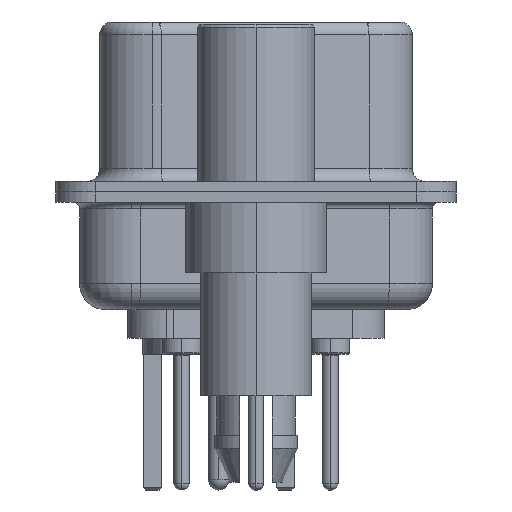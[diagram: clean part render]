
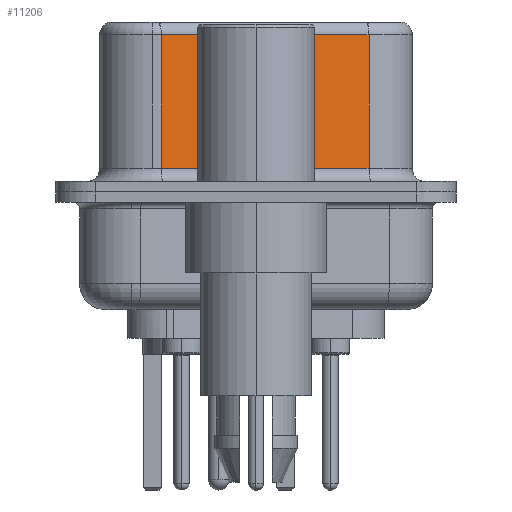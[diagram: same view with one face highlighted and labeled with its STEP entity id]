
A CAD part, left-side view. The second image highlights one B-rep face of the part: STEP entity #11206.
In plain terms, the highlighted planar face has unit normal (-0.985, -0.174, 0).
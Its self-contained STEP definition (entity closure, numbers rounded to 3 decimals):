
#1480 = ORIENTED_EDGE ( 'NONE', *, *, #23325, .T. ) ;
#1945 = VERTEX_POINT ( 'NONE', #15539 ) ;
#2792 = DIRECTION ( 'NONE',  ( 0.174, -0.985, 0. ) ) ;
#2866 = ORIENTED_EDGE ( 'NONE', *, *, #33034, .F. ) ;
#4109 = VERTEX_POINT ( 'NONE', #19650 ) ;
#4393 = CARTESIAN_POINT ( 'NONE',  ( 5.132, -4.322, 6.02 ) ) ;
#5450 = FACE_OUTER_BOUND ( 'NONE', #17898, .T. ) ;
#7857 = LINE ( 'NONE', #10828, #13479 ) ;
#8538 = DIRECTION ( 'NONE',  ( 0., 0., -1. ) ) ;
#8656 = CARTESIAN_POINT ( 'NONE',  ( 3.73, 3.628, 6.52 ) ) ;
#9259 = VECTOR ( 'NONE', #8538, 1000. ) ;
#9314 = VERTEX_POINT ( 'NONE', #12347 ) ;
#10828 = CARTESIAN_POINT ( 'NONE',  ( 5.132, -4.322, 0.9 ) ) ;
#11206 = ADVANCED_FACE ( 'NONE', ( #5450 ), #20425, .F. ) ;
#12347 = CARTESIAN_POINT ( 'NONE',  ( 3.73, 3.628, 0.9 ) ) ;
#12381 = CARTESIAN_POINT ( 'NONE',  ( 5.132, -4.322, 6.52 ) ) ;
#12497 = DIRECTION ( 'NONE',  ( 0., 0., -1. ) ) ;
#13479 = VECTOR ( 'NONE', #2792, 1000. ) ;
#15275 = VECTOR ( 'NONE', #12497, 1000. ) ;
#15323 = ORIENTED_EDGE ( 'NONE', *, *, #28274, .T. ) ;
#15539 = CARTESIAN_POINT ( 'NONE',  ( 5.132, -4.322, 0.9 ) ) ;
#16829 = LINE ( 'NONE', #4393, #22804 ) ;
#17898 = EDGE_LOOP ( 'NONE', ( #2866, #1480, #21370, #15323 ) ) ;
#19584 = LINE ( 'NONE', #8656, #9259 ) ;
#19650 = CARTESIAN_POINT ( 'NONE',  ( 3.73, 3.628, 6.02 ) ) ;
#20425 = PLANE ( 'NONE',  #24597 ) ;
#21370 = ORIENTED_EDGE ( 'NONE', *, *, #27093, .T. ) ;
#21708 = LINE ( 'NONE', #12381, #15275 ) ;
#22761 = CARTESIAN_POINT ( 'NONE',  ( 5.132, -4.322, 6.02 ) ) ;
#22804 = VECTOR ( 'NONE', #29597, 1000. ) ;
#23160 = CARTESIAN_POINT ( 'NONE',  ( 5.132, -4.322, 6.52 ) ) ;
#23325 = EDGE_CURVE ( 'NONE', #24907, #4109, #16829, .T. ) ;
#24597 = AXIS2_PLACEMENT_3D ( 'NONE', #23160, #34472, #26399 ) ;
#24907 = VERTEX_POINT ( 'NONE', #22761 ) ;
#26399 = DIRECTION ( 'NONE',  ( -0.174, 0.985, 0. ) ) ;
#27093 = EDGE_CURVE ( 'NONE', #4109, #9314, #19584, .T. ) ;
#28274 = EDGE_CURVE ( 'NONE', #9314, #1945, #7857, .T. ) ;
#29597 = DIRECTION ( 'NONE',  ( -0.174, 0.985, 0. ) ) ;
#33034 = EDGE_CURVE ( 'NONE', #24907, #1945, #21708, .T. ) ;
#34472 = DIRECTION ( 'NONE',  ( 0.985, 0.174, 0. ) ) ;
